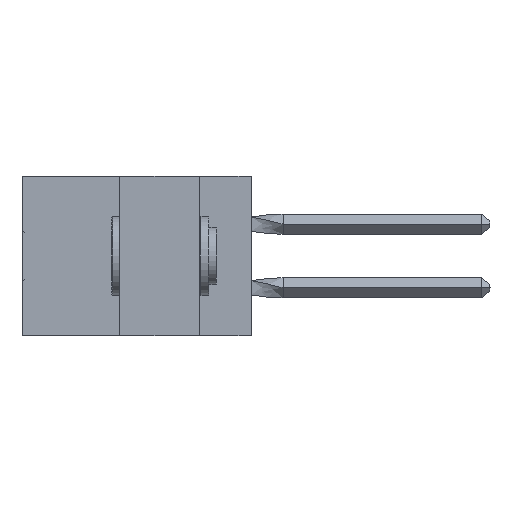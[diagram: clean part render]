
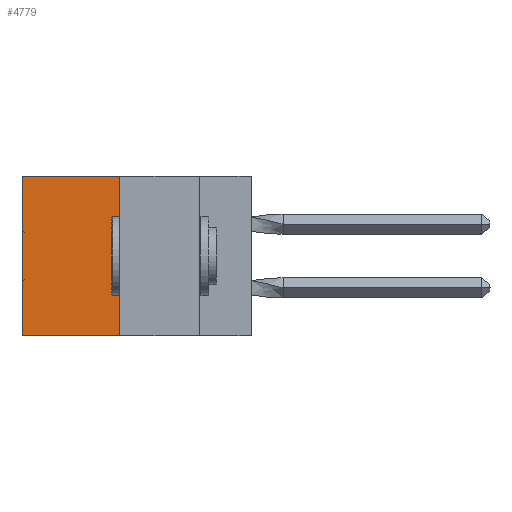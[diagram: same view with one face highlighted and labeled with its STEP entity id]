
A CAD part, left-side view. The second image highlights one B-rep face of the part: STEP entity #4779.
In plain terms, the highlighted planar face has unit normal (-1, 0, 0).
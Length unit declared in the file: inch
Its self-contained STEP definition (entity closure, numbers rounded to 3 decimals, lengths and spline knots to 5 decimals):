
#1822 = LINE ( 'NONE', #17157, #14781 ) ;
#3602 = LINE ( 'NONE', #43750, #20443 ) ;
#4779 = ADVANCED_FACE ( 'NONE', ( #47365 ), #43096, .F. ) ;
#6121 = DIRECTION ( 'NONE',  ( 0., 1., 0. ) ) ;
#7240 = CARTESIAN_POINT ( 'NONE',  ( 0.305, 0.72, -0.5 ) ) ;
#8113 = VERTEX_POINT ( 'NONE', #7240 ) ;
#8717 = CARTESIAN_POINT ( 'NONE',  ( 0.305, 0.413, 0. ) ) ;
#9140 = AXIS2_PLACEMENT_3D ( 'NONE', #34399, #26371, #27222 ) ;
#9520 = CARTESIAN_POINT ( 'NONE',  ( 0.305, 0.72, 0. ) ) ;
#9651 = EDGE_LOOP ( 'NONE', ( #13512, #46317, #24179, #45805 ) ) ;
#13512 = ORIENTED_EDGE ( 'NONE', *, *, #36646, .T. ) ;
#14781 = VECTOR ( 'NONE', #21820, 39.37008 ) ;
#17157 = CARTESIAN_POINT ( 'NONE',  ( 0.305, 0.413, -0.5 ) ) ;
#18903 = VECTOR ( 'NONE', #34878, 39.37008 ) ;
#19453 = VERTEX_POINT ( 'NONE', #8717 ) ;
#20443 = VECTOR ( 'NONE', #40501, 39.37008 ) ;
#21820 = DIRECTION ( 'NONE',  ( 0., 1., 0. ) ) ;
#23130 = CARTESIAN_POINT ( 'NONE',  ( 0.305, 0.413, 0. ) ) ;
#23425 = EDGE_CURVE ( 'NONE', #19453, #50645, #35540, .T. ) ;
#24179 = ORIENTED_EDGE ( 'NONE', *, *, #27802, .F. ) ;
#24666 = VECTOR ( 'NONE', #6121, 39.37008 ) ;
#26371 = DIRECTION ( 'NONE',  ( 1., 0., 0. ) ) ;
#27222 = DIRECTION ( 'NONE',  ( 0., 0., -1. ) ) ;
#27797 = VERTEX_POINT ( 'NONE', #38013 ) ;
#27802 = EDGE_CURVE ( 'NONE', #19453, #27797, #27970, .T. ) ;
#27970 = LINE ( 'NONE', #46289, #18903 ) ;
#34039 = EDGE_CURVE ( 'NONE', #27797, #8113, #1822, .T. ) ;
#34399 = CARTESIAN_POINT ( 'NONE',  ( 0.305, 0.413, -0.5 ) ) ;
#34878 = DIRECTION ( 'NONE',  ( 0., 0., -1. ) ) ;
#35540 = LINE ( 'NONE', #23130, #24666 ) ;
#36646 = EDGE_CURVE ( 'NONE', #50645, #8113, #3602, .T. ) ;
#38013 = CARTESIAN_POINT ( 'NONE',  ( 0.305, 0.413, -0.5 ) ) ;
#40501 = DIRECTION ( 'NONE',  ( 0., 0., -1. ) ) ;
#43096 = PLANE ( 'NONE',  #9140 ) ;
#43750 = CARTESIAN_POINT ( 'NONE',  ( 0.305, 0.72, -0.5 ) ) ;
#45805 = ORIENTED_EDGE ( 'NONE', *, *, #23425, .T. ) ;
#46289 = CARTESIAN_POINT ( 'NONE',  ( 0.305, 0.413, -0.5 ) ) ;
#46317 = ORIENTED_EDGE ( 'NONE', *, *, #34039, .F. ) ;
#47365 = FACE_OUTER_BOUND ( 'NONE', #9651, .T. ) ;
#50645 = VERTEX_POINT ( 'NONE', #9520 ) ;
